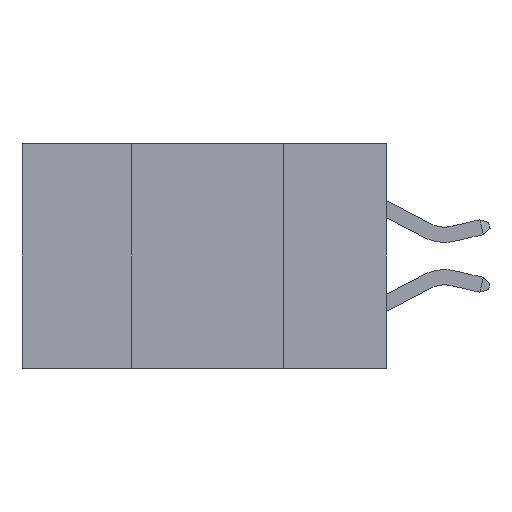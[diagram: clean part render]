
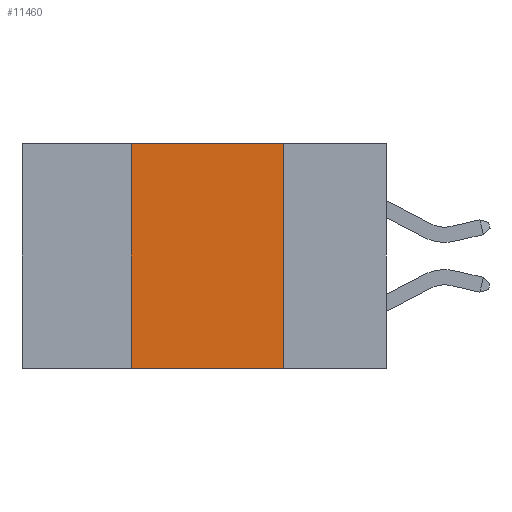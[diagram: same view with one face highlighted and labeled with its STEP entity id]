
A CAD part, left-side view. The second image highlights one B-rep face of the part: STEP entity #11460.
In plain terms, the highlighted planar face has unit normal (-1, 0, 0).
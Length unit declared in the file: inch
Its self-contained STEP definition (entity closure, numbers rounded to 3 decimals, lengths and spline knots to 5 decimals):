
#96 = CARTESIAN_POINT ( 'NONE',  ( 0., 0.6, -0.37 ) ) ;
#339 = EDGE_LOOP ( 'NONE', ( #17547, #2189, #9339, #3925 ) ) ;
#2189 = ORIENTED_EDGE ( 'NONE', *, *, #9538, .F. ) ;
#3690 = CARTESIAN_POINT ( 'NONE',  ( 0., 0.17, -0.37 ) ) ;
#3925 = ORIENTED_EDGE ( 'NONE', *, *, #17775, .T. ) ;
#4292 = VERTEX_POINT ( 'NONE', #3690 ) ;
#4317 = VERTEX_POINT ( 'NONE', #9716 ) ;
#5710 = PLANE ( 'NONE',  #18345 ) ;
#6403 = EDGE_CURVE ( 'NONE', #4317, #4292, #14093, .T. ) ;
#6829 = CARTESIAN_POINT ( 'NONE',  ( 0., 0.17, -0.37 ) ) ;
#7001 = DIRECTION ( 'NONE',  ( 0., -1., 0. ) ) ;
#7932 = DIRECTION ( 'NONE',  ( 0., -1., 0. ) ) ;
#8588 = DIRECTION ( 'NONE',  ( 0., 0., -1. ) ) ;
#9293 = CARTESIAN_POINT ( 'NONE',  ( 0., 0.42, 0. ) ) ;
#9339 = ORIENTED_EDGE ( 'NONE', *, *, #14307, .F. ) ;
#9359 = VECTOR ( 'NONE', #11139, 39.37008 ) ;
#9538 = EDGE_CURVE ( 'NONE', #12565, #4317, #11607, .T. ) ;
#9716 = CARTESIAN_POINT ( 'NONE',  ( 0., 0.17, 0. ) ) ;
#9964 = DIRECTION ( 'NONE',  ( 1., 0., 0. ) ) ;
#11139 = DIRECTION ( 'NONE',  ( 0., 0., -1. ) ) ;
#11460 = ADVANCED_FACE ( 'NONE', ( #16219 ), #5710, .F. ) ;
#11607 = LINE ( 'NONE', #19225, #16741 ) ;
#12565 = VERTEX_POINT ( 'NONE', #9293 ) ;
#13196 = CARTESIAN_POINT ( 'NONE',  ( 0., 0.42, -0.37 ) ) ;
#13543 = LINE ( 'NONE', #96, #16167 ) ;
#13655 = VERTEX_POINT ( 'NONE', #13196 ) ;
#14093 = LINE ( 'NONE', #6829, #9359 ) ;
#14307 = EDGE_CURVE ( 'NONE', #13655, #12565, #16568, .T. ) ;
#15111 = CARTESIAN_POINT ( 'NONE',  ( 0., 0.42, -0.37 ) ) ;
#15393 = DIRECTION ( 'NONE',  ( 0., 0., 1. ) ) ;
#16167 = VECTOR ( 'NONE', #7932, 39.37008 ) ;
#16219 = FACE_OUTER_BOUND ( 'NONE', #339, .T. ) ;
#16318 = CARTESIAN_POINT ( 'NONE',  ( 0., 0.6, 0. ) ) ;
#16486 = VECTOR ( 'NONE', #15393, 39.37008 ) ;
#16568 = LINE ( 'NONE', #15111, #16486 ) ;
#16741 = VECTOR ( 'NONE', #7001, 39.37008 ) ;
#17547 = ORIENTED_EDGE ( 'NONE', *, *, #6403, .F. ) ;
#17775 = EDGE_CURVE ( 'NONE', #13655, #4292, #13543, .T. ) ;
#18345 = AXIS2_PLACEMENT_3D ( 'NONE', #16318, #9964, #8588 ) ;
#19225 = CARTESIAN_POINT ( 'NONE',  ( 0., 0.6, 0. ) ) ;
